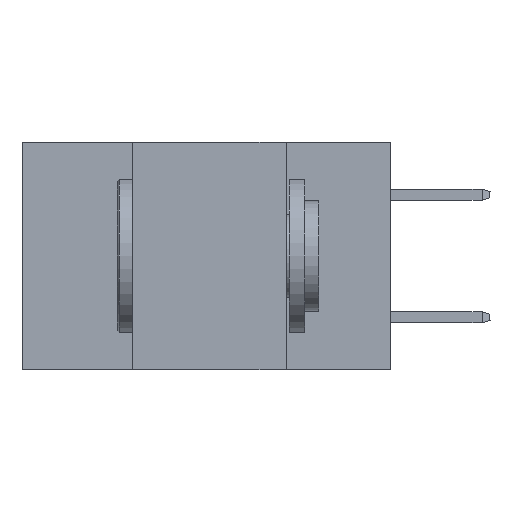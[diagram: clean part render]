
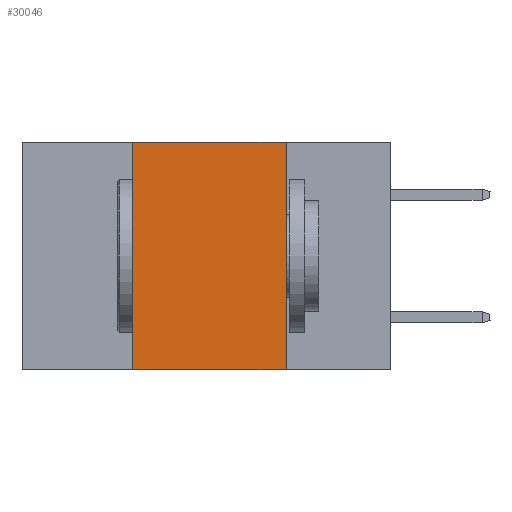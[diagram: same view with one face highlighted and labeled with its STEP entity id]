
A CAD part, left-side view. The second image highlights one B-rep face of the part: STEP entity #30046.
In plain terms, the highlighted planar face has unit normal (-1, 0, 0).
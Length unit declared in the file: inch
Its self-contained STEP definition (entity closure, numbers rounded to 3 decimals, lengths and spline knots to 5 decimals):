
#451 = AXIS2_PLACEMENT_3D ( 'NONE', #29898, #32338, #17456 ) ;
#1092 = ORIENTED_EDGE ( 'NONE', *, *, #5534, .F. ) ;
#1764 = VECTOR ( 'NONE', #10983, 39.37008 ) ;
#2156 = EDGE_CURVE ( 'NONE', #27635, #3076, #8584, .T. ) ;
#2586 = EDGE_CURVE ( 'NONE', #27635, #29506, #22611, .T. ) ;
#2682 = ORIENTED_EDGE ( 'NONE', *, *, #2586, .F. ) ;
#3076 = VERTEX_POINT ( 'NONE', #24265 ) ;
#4158 = VERTEX_POINT ( 'NONE', #19045 ) ;
#5446 = CARTESIAN_POINT ( 'NONE',  ( 0., 0.42, -0.37 ) ) ;
#5534 = EDGE_CURVE ( 'NONE', #29506, #4158, #6390, .T. ) ;
#6302 = CARTESIAN_POINT ( 'NONE',  ( 0., 0.17, 0. ) ) ;
#6390 = LINE ( 'NONE', #21256, #24832 ) ;
#6627 = LINE ( 'NONE', #6302, #25074 ) ;
#7084 = ORIENTED_EDGE ( 'NONE', *, *, #24527, .F. ) ;
#8062 = CARTESIAN_POINT ( 'NONE',  ( 0., 0.42, 0. ) ) ;
#8584 = LINE ( 'NONE', #12106, #1764 ) ;
#10983 = DIRECTION ( 'NONE',  ( 0., -1., 0. ) ) ;
#11329 = DIRECTION ( 'NONE',  ( 0., -1., 0. ) ) ;
#12106 = CARTESIAN_POINT ( 'NONE',  ( 0., 0.6, -0.37 ) ) ;
#12443 = PLANE ( 'NONE',  #451 ) ;
#13829 = DIRECTION ( 'NONE',  ( 0., 0., -1. ) ) ;
#16144 = ORIENTED_EDGE ( 'NONE', *, *, #2156, .T. ) ;
#17456 = DIRECTION ( 'NONE',  ( 0., 0., -1. ) ) ;
#19045 = CARTESIAN_POINT ( 'NONE',  ( 0., 0.17, 0. ) ) ;
#21256 = CARTESIAN_POINT ( 'NONE',  ( 0., 0.6, 0. ) ) ;
#22611 = LINE ( 'NONE', #25632, #30056 ) ;
#24265 = CARTESIAN_POINT ( 'NONE',  ( 0., 0.17, -0.37 ) ) ;
#24527 = EDGE_CURVE ( 'NONE', #4158, #3076, #6627, .T. ) ;
#24832 = VECTOR ( 'NONE', #11329, 39.37008 ) ;
#25074 = VECTOR ( 'NONE', #13829, 39.37008 ) ;
#25632 = CARTESIAN_POINT ( 'NONE',  ( 0., 0.42, 0. ) ) ;
#25932 = EDGE_LOOP ( 'NONE', ( #7084, #1092, #2682, #16144 ) ) ;
#27084 = DIRECTION ( 'NONE',  ( 0., 0., 1. ) ) ;
#27635 = VERTEX_POINT ( 'NONE', #5446 ) ;
#29506 = VERTEX_POINT ( 'NONE', #8062 ) ;
#29898 = CARTESIAN_POINT ( 'NONE',  ( 0., 0.6, 0. ) ) ;
#30046 = ADVANCED_FACE ( 'NONE', ( #30214 ), #12443, .F. ) ;
#30056 = VECTOR ( 'NONE', #27084, 39.37008 ) ;
#30214 = FACE_OUTER_BOUND ( 'NONE', #25932, .T. ) ;
#32338 = DIRECTION ( 'NONE',  ( 1., 0., 0. ) ) ;
